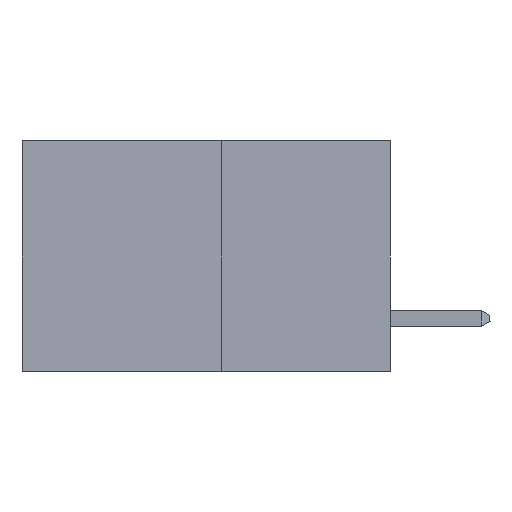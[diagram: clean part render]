
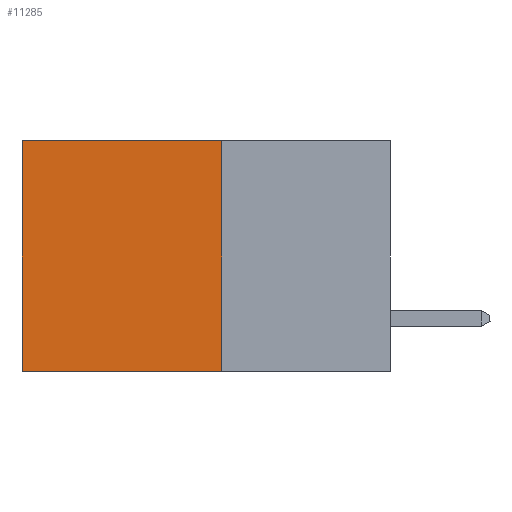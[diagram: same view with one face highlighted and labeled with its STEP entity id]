
A CAD part, left-side view. The second image highlights one B-rep face of the part: STEP entity #11285.
In plain terms, the highlighted planar face has unit normal (-1, 0, 0).
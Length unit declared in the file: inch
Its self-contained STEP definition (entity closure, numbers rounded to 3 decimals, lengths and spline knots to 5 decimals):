
#1576 = FACE_OUTER_BOUND ( 'NONE', #19822, .T. ) ;
#1906 = DIRECTION ( 'NONE',  ( 0., 0., -1. ) ) ;
#1969 = VECTOR ( 'NONE', #1906, 39.37008 ) ;
#2772 = DIRECTION ( 'NONE',  ( 0., 0., -1. ) ) ;
#3525 = LINE ( 'NONE', #18777, #1969 ) ;
#3881 = DIRECTION ( 'NONE',  ( 0., 0., -1. ) ) ;
#4051 = AXIS2_PLACEMENT_3D ( 'NONE', #9978, #17192, #2772 ) ;
#5117 = PLANE ( 'NONE',  #4051 ) ;
#8396 = CARTESIAN_POINT ( 'NONE',  ( 0.277, 0.59, 0. ) ) ;
#8830 = DIRECTION ( 'NONE',  ( 0., 1., 0. ) ) ;
#8925 = CARTESIAN_POINT ( 'NONE',  ( 0.277, 0.27, -0.37 ) ) ;
#9013 = LINE ( 'NONE', #26765, #27401 ) ;
#9978 = CARTESIAN_POINT ( 'NONE',  ( 0.277, 0.27, -0.37 ) ) ;
#10991 = CARTESIAN_POINT ( 'NONE',  ( 0.277, 0.27, 0. ) ) ;
#11079 = EDGE_CURVE ( 'NONE', #26912, #27545, #3525, .T. ) ;
#11285 = ADVANCED_FACE ( 'NONE', ( #1576 ), #5117, .F. ) ;
#11557 = VERTEX_POINT ( 'NONE', #10991 ) ;
#14690 = EDGE_CURVE ( 'NONE', #11557, #16885, #23992, .T. ) ;
#14844 = DIRECTION ( 'NONE',  ( 0., 1., 0. ) ) ;
#16885 = VERTEX_POINT ( 'NONE', #8925 ) ;
#16909 = VECTOR ( 'NONE', #3881, 39.37008 ) ;
#17192 = DIRECTION ( 'NONE',  ( 1., 0., 0. ) ) ;
#18443 = ORIENTED_EDGE ( 'NONE', *, *, #14690, .F. ) ;
#18777 = CARTESIAN_POINT ( 'NONE',  ( 0.277, 0.59, -0.37 ) ) ;
#19822 = EDGE_LOOP ( 'NONE', ( #24725, #21580, #18443, #25639 ) ) ;
#20377 = EDGE_CURVE ( 'NONE', #11557, #26912, #28035, .T. ) ;
#20712 = CARTESIAN_POINT ( 'NONE',  ( 0.277, 0.27, -0.37 ) ) ;
#20757 = CARTESIAN_POINT ( 'NONE',  ( 0.277, 0.27, 0. ) ) ;
#21580 = ORIENTED_EDGE ( 'NONE', *, *, #27980, .F. ) ;
#21657 = VECTOR ( 'NONE', #8830, 39.37008 ) ;
#23992 = LINE ( 'NONE', #20712, #16909 ) ;
#24725 = ORIENTED_EDGE ( 'NONE', *, *, #11079, .T. ) ;
#25639 = ORIENTED_EDGE ( 'NONE', *, *, #20377, .T. ) ;
#26765 = CARTESIAN_POINT ( 'NONE',  ( 0.277, 0.27, -0.37 ) ) ;
#26912 = VERTEX_POINT ( 'NONE', #8396 ) ;
#27401 = VECTOR ( 'NONE', #14844, 39.37008 ) ;
#27545 = VERTEX_POINT ( 'NONE', #27622 ) ;
#27622 = CARTESIAN_POINT ( 'NONE',  ( 0.277, 0.59, -0.37 ) ) ;
#27980 = EDGE_CURVE ( 'NONE', #16885, #27545, #9013, .T. ) ;
#28035 = LINE ( 'NONE', #20757, #21657 ) ;
